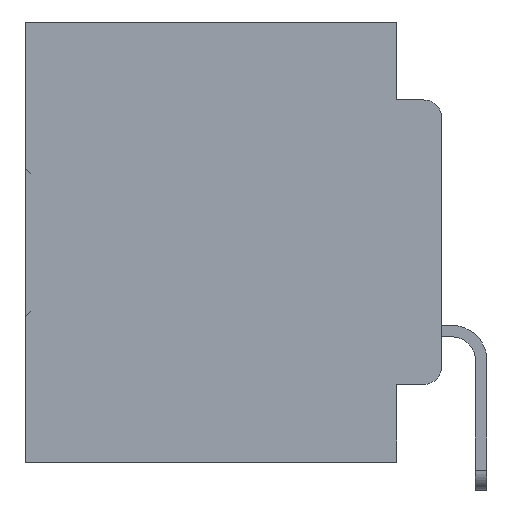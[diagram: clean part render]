
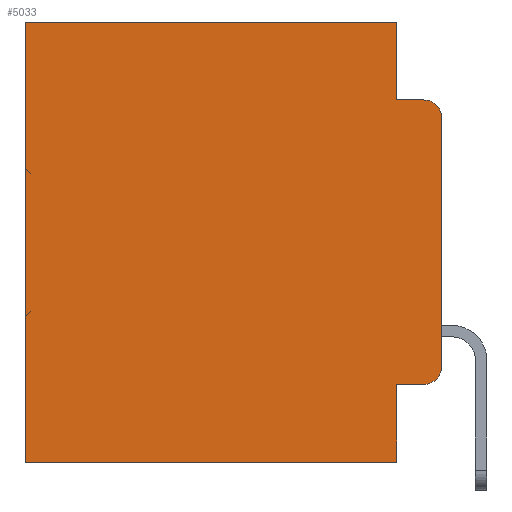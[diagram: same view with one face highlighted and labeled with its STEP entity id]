
A CAD part, left-side view. The second image highlights one B-rep face of the part: STEP entity #5033.
In plain terms, the highlighted planar face has unit normal (-1, 0, 0).
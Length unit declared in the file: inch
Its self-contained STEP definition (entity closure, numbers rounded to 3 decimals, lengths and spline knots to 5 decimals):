
#101 = LINE ( 'NONE', #24874, #21896 ) ;
#434 = CARTESIAN_POINT ( 'NONE',  ( 0.298, 0., -0.1085 ) ) ;
#1336 = EDGE_CURVE ( 'NONE', #22018, #16770, #28368, .T. ) ;
#1456 = VECTOR ( 'NONE', #17452, 39.37008 ) ;
#1524 = VECTOR ( 'NONE', #7057, 39.37008 ) ;
#1658 = VERTEX_POINT ( 'NONE', #33558 ) ;
#1733 = DIRECTION ( 'NONE',  ( 0., 0., -1. ) ) ;
#1929 = CARTESIAN_POINT ( 'NONE',  ( 0.298, 0., 0. ) ) ;
#2393 = LINE ( 'NONE', #30837, #1456 ) ;
#2666 = CARTESIAN_POINT ( 'NONE',  ( 0.298, 0., -0.3915 ) ) ;
#2801 = VERTEX_POINT ( 'NONE', #19472 ) ;
#3244 = FACE_OUTER_BOUND ( 'NONE', #13449, .T. ) ;
#4191 = CARTESIAN_POINT ( 'NONE',  ( 0.298, 0., -0.5 ) ) ;
#4197 = EDGE_CURVE ( 'NONE', #10340, #17898, #20584, .T. ) ;
#4489 = DIRECTION ( 'NONE',  ( 0., 0., -1. ) ) ;
#5033 = ADVANCED_FACE ( 'NONE', ( #3244 ), #19354, .F. ) ;
#5393 = VECTOR ( 'NONE', #24368, 39.37008 ) ;
#6168 = AXIS2_PLACEMENT_3D ( 'NONE', #7999, #27319, #10986 ) ;
#6794 = VECTOR ( 'NONE', #1733, 39.37008 ) ;
#6952 = VERTEX_POINT ( 'NONE', #2666 ) ;
#7034 = CARTESIAN_POINT ( 'NONE',  ( 0.298, 0.02, -0.1085 ) ) ;
#7057 = DIRECTION ( 'NONE',  ( 0., 1., 0. ) ) ;
#7133 = ORIENTED_EDGE ( 'NONE', *, *, #22984, .F. ) ;
#7339 = VERTEX_POINT ( 'NONE', #20348 ) ;
#7892 = CARTESIAN_POINT ( 'NONE',  ( 0.298, 0., 0. ) ) ;
#7999 = CARTESIAN_POINT ( 'NONE',  ( 0.298, 0.02, -0.3915 ) ) ;
#8233 = VERTEX_POINT ( 'NONE', #34545 ) ;
#8423 = CARTESIAN_POINT ( 'NONE',  ( 0.298, 0.051, -0.5 ) ) ;
#8541 = CIRCLE ( 'NONE', #6168, 0.02 ) ;
#8980 = ORIENTED_EDGE ( 'NONE', *, *, #34182, .T. ) ;
#9417 = ORIENTED_EDGE ( 'NONE', *, *, #13904, .F. ) ;
#9897 = CARTESIAN_POINT ( 'NONE',  ( 0.298, 0.051, 0. ) ) ;
#10007 = DIRECTION ( 'NONE',  ( 0., 0., -1. ) ) ;
#10340 = VERTEX_POINT ( 'NONE', #19048 ) ;
#10345 = ORIENTED_EDGE ( 'NONE', *, *, #24773, .T. ) ;
#10986 = DIRECTION ( 'NONE',  ( 0., 0., -1. ) ) ;
#11458 = DIRECTION ( 'NONE',  ( 0., -1., 0. ) ) ;
#11467 = LINE ( 'NONE', #18950, #32904 ) ;
#12014 = EDGE_CURVE ( 'NONE', #16770, #1658, #101, .T. ) ;
#13449 = EDGE_LOOP ( 'NONE', ( #19514, #10345, #7133, #9417, #21316, #28814, #19138, #22039, #8980, #14412 ) ) ;
#13904 = EDGE_CURVE ( 'NONE', #22018, #8233, #11467, .T. ) ;
#14412 = ORIENTED_EDGE ( 'NONE', *, *, #21851, .T. ) ;
#14475 = CARTESIAN_POINT ( 'NONE',  ( 0.298, 0.051, 0. ) ) ;
#14529 = LINE ( 'NONE', #16152, #6794 ) ;
#14656 = VERTEX_POINT ( 'NONE', #434 ) ;
#14970 = VECTOR ( 'NONE', #11458, 39.37008 ) ;
#15686 = DIRECTION ( 'NONE',  ( 1., 0., 0. ) ) ;
#15837 = LINE ( 'NONE', #24952, #14970 ) ;
#16027 = LINE ( 'NONE', #4191, #1524 ) ;
#16152 = CARTESIAN_POINT ( 'NONE',  ( 0.298, 0., 0. ) ) ;
#16770 = VERTEX_POINT ( 'NONE', #32560 ) ;
#17452 = DIRECTION ( 'NONE',  ( 0., -1., 0. ) ) ;
#17898 = VERTEX_POINT ( 'NONE', #8423 ) ;
#18916 = VECTOR ( 'NONE', #29018, 39.37008 ) ;
#18950 = CARTESIAN_POINT ( 'NONE',  ( 0.298, 0.051, 0. ) ) ;
#19048 = CARTESIAN_POINT ( 'NONE',  ( 0.298, 0.051, -0.4115 ) ) ;
#19138 = ORIENTED_EDGE ( 'NONE', *, *, #29317, .F. ) ;
#19354 = PLANE ( 'NONE',  #22705 ) ;
#19472 = CARTESIAN_POINT ( 'NONE',  ( 0.298, 0.02, -0.0885 ) ) ;
#19514 = ORIENTED_EDGE ( 'NONE', *, *, #23037, .F. ) ;
#20348 = CARTESIAN_POINT ( 'NONE',  ( 0.298, 0.02, -0.4115 ) ) ;
#20584 = LINE ( 'NONE', #9897, #18916 ) ;
#21316 = ORIENTED_EDGE ( 'NONE', *, *, #1336, .T. ) ;
#21609 = DIRECTION ( 'NONE',  ( 0., 0., -1. ) ) ;
#21851 = EDGE_CURVE ( 'NONE', #7339, #6952, #8541, .T. ) ;
#21896 = VECTOR ( 'NONE', #27665, 39.37008 ) ;
#22018 = VERTEX_POINT ( 'NONE', #14475 ) ;
#22039 = ORIENTED_EDGE ( 'NONE', *, *, #4197, .F. ) ;
#22705 = AXIS2_PLACEMENT_3D ( 'NONE', #7892, #15686, #4489 ) ;
#22984 = EDGE_CURVE ( 'NONE', #8233, #2801, #15837, .T. ) ;
#23037 = EDGE_CURVE ( 'NONE', #14656, #6952, #14529, .T. ) ;
#23559 = AXIS2_PLACEMENT_3D ( 'NONE', #7034, #26447, #10007 ) ;
#24368 = DIRECTION ( 'NONE',  ( 0., 1., 0. ) ) ;
#24773 = EDGE_CURVE ( 'NONE', #14656, #2801, #25422, .T. ) ;
#24874 = CARTESIAN_POINT ( 'NONE',  ( 0.298, 0.473, 0. ) ) ;
#24952 = CARTESIAN_POINT ( 'NONE',  ( 0.298, 0.051, -0.0885 ) ) ;
#25422 = CIRCLE ( 'NONE', #23559, 0.02 ) ;
#26447 = DIRECTION ( 'NONE',  ( -1., 0., 0. ) ) ;
#27319 = DIRECTION ( 'NONE',  ( -1., 0., 0. ) ) ;
#27665 = DIRECTION ( 'NONE',  ( 0., 0., -1. ) ) ;
#28368 = LINE ( 'NONE', #1929, #5393 ) ;
#28814 = ORIENTED_EDGE ( 'NONE', *, *, #12014, .T. ) ;
#29018 = DIRECTION ( 'NONE',  ( 0., 0., -1. ) ) ;
#29317 = EDGE_CURVE ( 'NONE', #17898, #1658, #16027, .T. ) ;
#30837 = CARTESIAN_POINT ( 'NONE',  ( 0.298, 0.051, -0.4115 ) ) ;
#32560 = CARTESIAN_POINT ( 'NONE',  ( 0.298, 0.473, 0. ) ) ;
#32904 = VECTOR ( 'NONE', #21609, 39.37008 ) ;
#33558 = CARTESIAN_POINT ( 'NONE',  ( 0.298, 0.473, -0.5 ) ) ;
#34182 = EDGE_CURVE ( 'NONE', #10340, #7339, #2393, .T. ) ;
#34545 = CARTESIAN_POINT ( 'NONE',  ( 0.298, 0.051, -0.0885 ) ) ;
